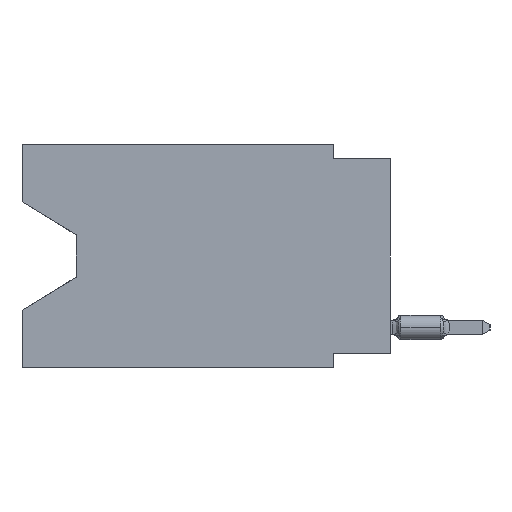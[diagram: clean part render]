
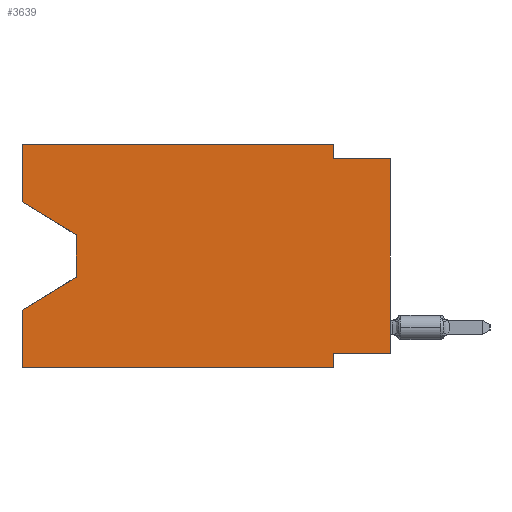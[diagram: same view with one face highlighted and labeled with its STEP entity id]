
A CAD part, left-side view. The second image highlights one B-rep face of the part: STEP entity #3639.
In plain terms, the highlighted planar face has unit normal (-1, 0, 0).
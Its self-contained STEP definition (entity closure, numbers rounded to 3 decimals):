
#754 = VECTOR ( 'NONE', #26916, 1000. ) ;
#1543 = DIRECTION ( 'NONE',  ( 0., 0., 1. ) ) ;
#2864 = VERTEX_POINT ( 'NONE', #25407 ) ;
#3478 = CARTESIAN_POINT ( 'NONE',  ( 0., 2.54, 0. ) ) ;
#3639 = ADVANCED_FACE ( 'NONE', ( #52151 ), #15574, .F. ) ;
#3819 = ORIENTED_EDGE ( 'NONE', *, *, #31856, .F. ) ;
#4384 = VERTEX_POINT ( 'NONE', #32880 ) ;
#5665 = EDGE_CURVE ( 'NONE', #61906, #22788, #38333, .T. ) ;
#5755 = DIRECTION ( 'NONE',  ( 0., 1., 0. ) ) ;
#6538 = VERTEX_POINT ( 'NONE', #61302 ) ;
#7273 = VERTEX_POINT ( 'NONE', #7507 ) ;
#7449 = VECTOR ( 'NONE', #41194, 1000. ) ;
#7507 = CARTESIAN_POINT ( 'NONE',  ( 0., 16.383, 0. ) ) ;
#8470 = LINE ( 'NONE', #13593, #14048 ) ;
#10540 = EDGE_CURVE ( 'NONE', #56718, #7273, #67011, .T. ) ;
#11128 = CARTESIAN_POINT ( 'NONE',  ( 0., 0., -0.635 ) ) ;
#12369 = DIRECTION ( 'NONE',  ( 0., -1., 0. ) ) ;
#12896 = ORIENTED_EDGE ( 'NONE', *, *, #60211, .F. ) ;
#13593 = CARTESIAN_POINT ( 'NONE',  ( 0., 16.383, 0. ) ) ;
#13762 = LINE ( 'NONE', #29816, #53521 ) ;
#14048 = VECTOR ( 'NONE', #29299, 1000. ) ;
#14610 = VECTOR ( 'NONE', #20180, 1000. ) ;
#15211 = VECTOR ( 'NONE', #58281, 1000. ) ;
#15574 = PLANE ( 'NONE',  #22808 ) ;
#16343 = CARTESIAN_POINT ( 'NONE',  ( 0., 0., -9.271 ) ) ;
#16603 = VECTOR ( 'NONE', #12369, 1000. ) ;
#16660 = CARTESIAN_POINT ( 'NONE',  ( 0., 0., 0. ) ) ;
#17898 = EDGE_CURVE ( 'NONE', #32347, #19162, #13762, .T. ) ;
#19162 = VERTEX_POINT ( 'NONE', #59955 ) ;
#19228 = ORIENTED_EDGE ( 'NONE', *, *, #5665, .T. ) ;
#20173 = ORIENTED_EDGE ( 'NONE', *, *, #17898, .T. ) ;
#20180 = DIRECTION ( 'NONE',  ( 0., 0., 1. ) ) ;
#22788 = VERTEX_POINT ( 'NONE', #26140 ) ;
#22808 = AXIS2_PLACEMENT_3D ( 'NONE', #41887, #36082, #56935 ) ;
#22999 = EDGE_LOOP ( 'NONE', ( #61353, #45124, #20173, #24684, #19228, #31240, #40146, #65326, #12896, #36838, #3819, #24262 ) ) ;
#24262 = ORIENTED_EDGE ( 'NONE', *, *, #10540, .F. ) ;
#24684 = ORIENTED_EDGE ( 'NONE', *, *, #53194, .F. ) ;
#24793 = CARTESIAN_POINT ( 'NONE',  ( 0., 13.97, -4.013 ) ) ;
#25107 = CARTESIAN_POINT ( 'NONE',  ( 0., 16.383, -9.906 ) ) ;
#25407 = CARTESIAN_POINT ( 'NONE',  ( 0., 0., -0.635 ) ) ;
#26140 = CARTESIAN_POINT ( 'NONE',  ( 0., 2.54, -9.906 ) ) ;
#26916 = DIRECTION ( 'NONE',  ( 0., 0., 1. ) ) ;
#27032 = VERTEX_POINT ( 'NONE', #35313 ) ;
#27051 = CARTESIAN_POINT ( 'NONE',  ( 0., 2.54, -0.635 ) ) ;
#27827 = EDGE_CURVE ( 'NONE', #6538, #22788, #32788, .T. ) ;
#29275 = VECTOR ( 'NONE', #5755, 1000. ) ;
#29299 = DIRECTION ( 'NONE',  ( 0., -1., 0. ) ) ;
#29529 = EDGE_CURVE ( 'NONE', #4384, #2864, #48116, .T. ) ;
#29816 = CARTESIAN_POINT ( 'NONE',  ( 0., 13.97, -5.893 ) ) ;
#30134 = EDGE_CURVE ( 'NONE', #46523, #50932, #34574, .T. ) ;
#30788 = EDGE_CURVE ( 'NONE', #4384, #6538, #63148, .T. ) ;
#31240 = ORIENTED_EDGE ( 'NONE', *, *, #27827, .F. ) ;
#31856 = EDGE_CURVE ( 'NONE', #7273, #46523, #8470, .T. ) ;
#31969 = LINE ( 'NONE', #47361, #47842 ) ;
#32347 = VERTEX_POINT ( 'NONE', #66468 ) ;
#32788 = LINE ( 'NONE', #43732, #36740 ) ;
#32880 = CARTESIAN_POINT ( 'NONE',  ( 0., 0., -9.271 ) ) ;
#34574 = LINE ( 'NONE', #3478, #37900 ) ;
#35313 = CARTESIAN_POINT ( 'NONE',  ( 0., 13.97, -4.013 ) ) ;
#36082 = DIRECTION ( 'NONE',  ( 1., 0., 0. ) ) ;
#36740 = VECTOR ( 'NONE', #53645, 1000. ) ;
#36838 = ORIENTED_EDGE ( 'NONE', *, *, #30134, .F. ) ;
#37900 = VECTOR ( 'NONE', #49972, 1000. ) ;
#38333 = LINE ( 'NONE', #59176, #16603 ) ;
#40146 = ORIENTED_EDGE ( 'NONE', *, *, #30788, .F. ) ;
#41193 = CARTESIAN_POINT ( 'NONE',  ( 0., 2.54, 0. ) ) ;
#41194 = DIRECTION ( 'NONE',  ( 0., 0., -1. ) ) ;
#41887 = CARTESIAN_POINT ( 'NONE',  ( 0., 16.383, 0. ) ) ;
#42896 = LINE ( 'NONE', #11128, #15211 ) ;
#43732 = CARTESIAN_POINT ( 'NONE',  ( 0., 2.54, -9.906 ) ) ;
#45124 = ORIENTED_EDGE ( 'NONE', *, *, #51872, .T. ) ;
#46523 = VERTEX_POINT ( 'NONE', #41193 ) ;
#47361 = CARTESIAN_POINT ( 'NONE',  ( 0., 16.383, 0. ) ) ;
#47842 = VECTOR ( 'NONE', #1543, 1000. ) ;
#48116 = LINE ( 'NONE', #16660, #754 ) ;
#49061 = CARTESIAN_POINT ( 'NONE',  ( 0., 16.383, -2.546 ) ) ;
#49972 = DIRECTION ( 'NONE',  ( 0., 0., -1. ) ) ;
#50334 = DIRECTION ( 'NONE',  ( 0., 0.855, -0.519 ) ) ;
#50625 = CARTESIAN_POINT ( 'NONE',  ( 0., 16.383, 0. ) ) ;
#50932 = VERTEX_POINT ( 'NONE', #27051 ) ;
#51872 = EDGE_CURVE ( 'NONE', #27032, #32347, #62029, .T. ) ;
#52151 = FACE_OUTER_BOUND ( 'NONE', #22999, .T. ) ;
#53194 = EDGE_CURVE ( 'NONE', #61906, #19162, #31969, .T. ) ;
#53521 = VECTOR ( 'NONE', #50334, 1000. ) ;
#53645 = DIRECTION ( 'NONE',  ( 0., 0., -1. ) ) ;
#54864 = EDGE_CURVE ( 'NONE', #56718, #27032, #57936, .T. ) ;
#56718 = VERTEX_POINT ( 'NONE', #49061 ) ;
#56935 = DIRECTION ( 'NONE',  ( 0., 0., -1. ) ) ;
#57936 = LINE ( 'NONE', #66938, #62217 ) ;
#58281 = DIRECTION ( 'NONE',  ( 0., -1., 0. ) ) ;
#59176 = CARTESIAN_POINT ( 'NONE',  ( 0., 16.383, -9.906 ) ) ;
#59955 = CARTESIAN_POINT ( 'NONE',  ( 0., 16.383, -7.36 ) ) ;
#60211 = EDGE_CURVE ( 'NONE', #50932, #2864, #42896, .T. ) ;
#61302 = CARTESIAN_POINT ( 'NONE',  ( 0., 2.54, -9.271 ) ) ;
#61353 = ORIENTED_EDGE ( 'NONE', *, *, #54864, .T. ) ;
#61906 = VERTEX_POINT ( 'NONE', #25107 ) ;
#62029 = LINE ( 'NONE', #24793, #7449 ) ;
#62217 = VECTOR ( 'NONE', #63048, 1000. ) ;
#63048 = DIRECTION ( 'NONE',  ( 0., -0.855, -0.519 ) ) ;
#63148 = LINE ( 'NONE', #16343, #29275 ) ;
#65326 = ORIENTED_EDGE ( 'NONE', *, *, #29529, .T. ) ;
#66468 = CARTESIAN_POINT ( 'NONE',  ( 0., 13.97, -5.893 ) ) ;
#66938 = CARTESIAN_POINT ( 'NONE',  ( 0., 16.383, -2.546 ) ) ;
#67011 = LINE ( 'NONE', #50625, #14610 ) ;
